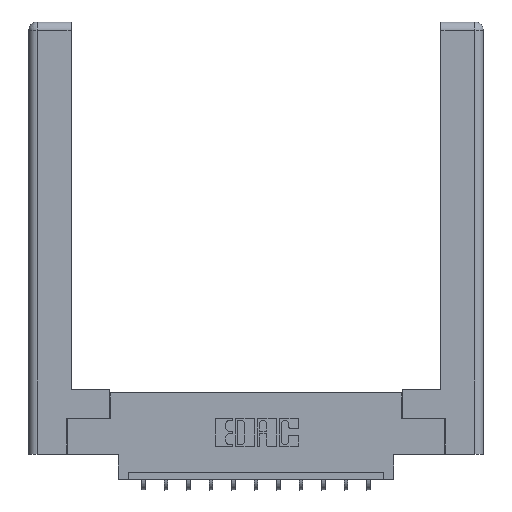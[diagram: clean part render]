
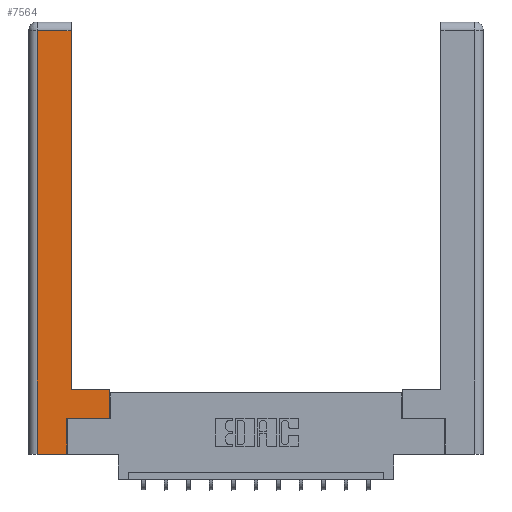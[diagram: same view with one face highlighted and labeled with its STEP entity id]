
A CAD part, top view. The second image highlights one B-rep face of the part: STEP entity #7564.
In plain terms, the highlighted planar face has unit normal (0, 0, 1).
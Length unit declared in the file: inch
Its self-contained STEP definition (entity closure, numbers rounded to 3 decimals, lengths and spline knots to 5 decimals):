
#40 = ORIENTED_EDGE ( 'NONE', *, *, #2203, .T. ) ;
#74 = CARTESIAN_POINT ( 'NONE',  ( 0.0615, 2.94, 0. ) ) ;
#736 = CARTESIAN_POINT ( 'NONE',  ( 0.0615, 0., 0. ) ) ;
#752 = CARTESIAN_POINT ( 'NONE',  ( 0.265, 0.245, 0. ) ) ;
#1036 = CARTESIAN_POINT ( 'NONE',  ( 0.565, 0.245, 0. ) ) ;
#1558 = CARTESIAN_POINT ( 'NONE',  ( 0.565, 0.45, 0. ) ) ;
#2168 = LINE ( 'NONE', #752, #10851 ) ;
#2203 = EDGE_CURVE ( 'NONE', #7719, #5001, #6950, .T. ) ;
#2291 = ORIENTED_EDGE ( 'NONE', *, *, #11670, .T. ) ;
#2427 = LINE ( 'NONE', #7676, #14391 ) ;
#2599 = VECTOR ( 'NONE', #11900, 39.37008 ) ;
#3986 = FACE_OUTER_BOUND ( 'NONE', #13995, .T. ) ;
#4283 = VERTEX_POINT ( 'NONE', #7123 ) ;
#4390 = PLANE ( 'NONE',  #11101 ) ;
#4396 = EDGE_CURVE ( 'NONE', #14674, #5458, #7699, .T. ) ;
#4583 = CARTESIAN_POINT ( 'NONE',  ( 0.265, 0., 0. ) ) ;
#4795 = EDGE_CURVE ( 'NONE', #11044, #4283, #2427, .T. ) ;
#4938 = EDGE_CURVE ( 'NONE', #5001, #14674, #12768, .T. ) ;
#4950 = LINE ( 'NONE', #1036, #7698 ) ;
#5001 = VERTEX_POINT ( 'NONE', #74 ) ;
#5033 = EDGE_CURVE ( 'NONE', #11904, #9911, #4950, .T. ) ;
#5458 = VERTEX_POINT ( 'NONE', #4583 ) ;
#5475 = DIRECTION ( 'NONE',  ( -1., 0., 0. ) ) ;
#5613 = VECTOR ( 'NONE', #6083, 39.37008 ) ;
#5750 = LINE ( 'NONE', #9361, #10648 ) ;
#6083 = DIRECTION ( 'NONE',  ( 0., 1., 0. ) ) ;
#6686 = ORIENTED_EDGE ( 'NONE', *, *, #4795, .T. ) ;
#6732 = CARTESIAN_POINT ( 'NONE',  ( 0.565, 0.45, 0. ) ) ;
#6940 = DIRECTION ( 'NONE',  ( -1., 0., 0. ) ) ;
#6950 = LINE ( 'NONE', #13646, #8400 ) ;
#6989 = DIRECTION ( 'NONE',  ( 0., 1., 0. ) ) ;
#7054 = CARTESIAN_POINT ( 'NONE',  ( 0.265, 0.245, 0. ) ) ;
#7123 = CARTESIAN_POINT ( 'NONE',  ( 0.295, 0.45, 0. ) ) ;
#7156 = ORIENTED_EDGE ( 'NONE', *, *, #5033, .T. ) ;
#7564 = ADVANCED_FACE ( 'NONE', ( #3986 ), #4390, .F. ) ;
#7676 = CARTESIAN_POINT ( 'NONE',  ( 0.295, 0.45, 0. ) ) ;
#7698 = VECTOR ( 'NONE', #12766, 39.37008 ) ;
#7699 = LINE ( 'NONE', #14013, #11107 ) ;
#7719 = VERTEX_POINT ( 'NONE', #11677 ) ;
#8095 = CARTESIAN_POINT ( 'NONE',  ( 0.565, 0.245, 0. ) ) ;
#8196 = CARTESIAN_POINT ( 'NONE',  ( 0.0615, 0., 0. ) ) ;
#8400 = VECTOR ( 'NONE', #5475, 39.37008 ) ;
#9361 = CARTESIAN_POINT ( 'NONE',  ( 0.295, 3., 0. ) ) ;
#9484 = EDGE_CURVE ( 'NONE', #4283, #7719, #5750, .T. ) ;
#9911 = VERTEX_POINT ( 'NONE', #8095 ) ;
#10648 = VECTOR ( 'NONE', #6989, 39.37008 ) ;
#10851 = VECTOR ( 'NONE', #12333, 39.37008 ) ;
#11044 = VERTEX_POINT ( 'NONE', #6732 ) ;
#11101 = AXIS2_PLACEMENT_3D ( 'NONE', #11529, #13865, #6940 ) ;
#11107 = VECTOR ( 'NONE', #13291, 39.37008 ) ;
#11414 = EDGE_CURVE ( 'NONE', #9911, #11044, #12139, .T. ) ;
#11529 = CARTESIAN_POINT ( 'NONE',  ( 0., 0., 0. ) ) ;
#11670 = EDGE_CURVE ( 'NONE', #5458, #11904, #2168, .T. ) ;
#11677 = CARTESIAN_POINT ( 'NONE',  ( 0.295, 2.94, 0. ) ) ;
#11900 = DIRECTION ( 'NONE',  ( 0., -1., 0. ) ) ;
#11904 = VERTEX_POINT ( 'NONE', #7054 ) ;
#12128 = ORIENTED_EDGE ( 'NONE', *, *, #9484, .T. ) ;
#12139 = LINE ( 'NONE', #1558, #5613 ) ;
#12333 = DIRECTION ( 'NONE',  ( 0., 1., 0. ) ) ;
#12766 = DIRECTION ( 'NONE',  ( 1., 0., 0. ) ) ;
#12768 = LINE ( 'NONE', #8196, #2599 ) ;
#13291 = DIRECTION ( 'NONE',  ( 1., 0., 0. ) ) ;
#13646 = CARTESIAN_POINT ( 'NONE',  ( 0.0615, 2.94, 0. ) ) ;
#13700 = ORIENTED_EDGE ( 'NONE', *, *, #4938, .T. ) ;
#13865 = DIRECTION ( 'NONE',  ( 0., 0., -1. ) ) ;
#13995 = EDGE_LOOP ( 'NONE', ( #12128, #40, #13700, #14099, #2291, #7156, #14490, #6686 ) ) ;
#14013 = CARTESIAN_POINT ( 'NONE',  ( 0.265, 0., 0. ) ) ;
#14099 = ORIENTED_EDGE ( 'NONE', *, *, #4396, .T. ) ;
#14391 = VECTOR ( 'NONE', #14708, 39.37008 ) ;
#14490 = ORIENTED_EDGE ( 'NONE', *, *, #11414, .T. ) ;
#14674 = VERTEX_POINT ( 'NONE', #736 ) ;
#14708 = DIRECTION ( 'NONE',  ( -1., 0., 0. ) ) ;
